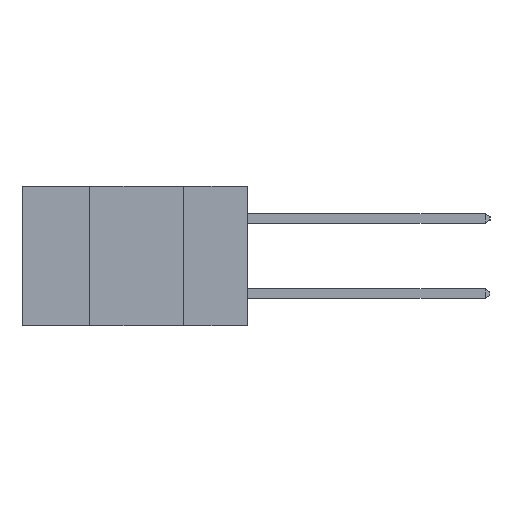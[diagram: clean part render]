
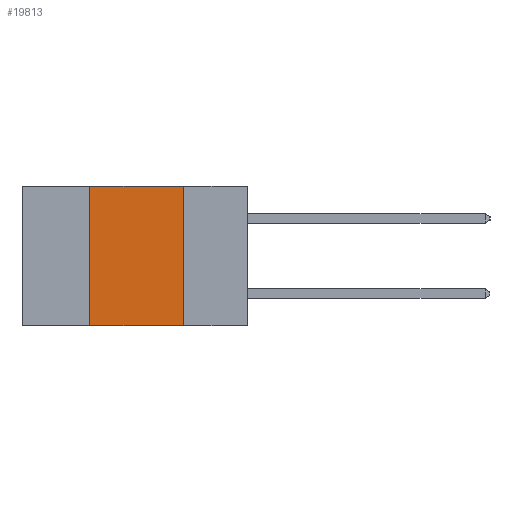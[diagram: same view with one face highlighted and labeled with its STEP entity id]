
A CAD part, left-side view. The second image highlights one B-rep face of the part: STEP entity #19813.
In plain terms, the highlighted planar face has unit normal (-1, 0, 0).
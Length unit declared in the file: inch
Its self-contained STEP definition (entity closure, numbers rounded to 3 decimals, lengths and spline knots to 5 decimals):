
#892 = VECTOR ( 'NONE', #26507, 39.37008 ) ;
#1786 = VERTEX_POINT ( 'NONE', #11524 ) ;
#2100 = DIRECTION ( 'NONE',  ( 0., -1., 0. ) ) ;
#2844 = EDGE_CURVE ( 'NONE', #1786, #5355, #17158, .T. ) ;
#3827 = CARTESIAN_POINT ( 'NONE',  ( 0., 0.6, 0. ) ) ;
#4399 = ORIENTED_EDGE ( 'NONE', *, *, #22895, .F. ) ;
#5173 = LINE ( 'NONE', #23061, #10141 ) ;
#5355 = VERTEX_POINT ( 'NONE', #24916 ) ;
#5968 = DIRECTION ( 'NONE',  ( 0., 0., -1. ) ) ;
#6375 = LINE ( 'NONE', #12646, #11326 ) ;
#7474 = VERTEX_POINT ( 'NONE', #24895 ) ;
#7649 = LINE ( 'NONE', #13156, #18121 ) ;
#9368 = ORIENTED_EDGE ( 'NONE', *, *, #14223, .T. ) ;
#10141 = VECTOR ( 'NONE', #2100, 39.37008 ) ;
#11326 = VECTOR ( 'NONE', #22995, 39.37008 ) ;
#11524 = CARTESIAN_POINT ( 'NONE',  ( 0., 0.17, 0. ) ) ;
#12646 = CARTESIAN_POINT ( 'NONE',  ( 0., 0.6, 0. ) ) ;
#13156 = CARTESIAN_POINT ( 'NONE',  ( 0., 0.42, -0.37 ) ) ;
#14223 = EDGE_CURVE ( 'NONE', #15742, #5355, #5173, .T. ) ;
#15251 = DIRECTION ( 'NONE',  ( 0., 0., 1. ) ) ;
#15742 = VERTEX_POINT ( 'NONE', #19916 ) ;
#17158 = LINE ( 'NONE', #25429, #892 ) ;
#17643 = ORIENTED_EDGE ( 'NONE', *, *, #23748, .F. ) ;
#18060 = EDGE_LOOP ( 'NONE', ( #24440, #4399, #17643, #9368 ) ) ;
#18121 = VECTOR ( 'NONE', #15251, 39.37008 ) ;
#18528 = DIRECTION ( 'NONE',  ( 1., 0., 0. ) ) ;
#19813 = ADVANCED_FACE ( 'NONE', ( #26217 ), #20540, .F. ) ;
#19916 = CARTESIAN_POINT ( 'NONE',  ( 0., 0.42, -0.37 ) ) ;
#20540 = PLANE ( 'NONE',  #25870 ) ;
#22895 = EDGE_CURVE ( 'NONE', #7474, #1786, #6375, .T. ) ;
#22995 = DIRECTION ( 'NONE',  ( 0., -1., 0. ) ) ;
#23061 = CARTESIAN_POINT ( 'NONE',  ( 0., 0.6, -0.37 ) ) ;
#23748 = EDGE_CURVE ( 'NONE', #15742, #7474, #7649, .T. ) ;
#24440 = ORIENTED_EDGE ( 'NONE', *, *, #2844, .F. ) ;
#24895 = CARTESIAN_POINT ( 'NONE',  ( 0., 0.42, 0. ) ) ;
#24916 = CARTESIAN_POINT ( 'NONE',  ( 0., 0.17, -0.37 ) ) ;
#25429 = CARTESIAN_POINT ( 'NONE',  ( 0., 0.17, -0.37 ) ) ;
#25870 = AXIS2_PLACEMENT_3D ( 'NONE', #3827, #18528, #5968 ) ;
#26217 = FACE_OUTER_BOUND ( 'NONE', #18060, .T. ) ;
#26507 = DIRECTION ( 'NONE',  ( 0., 0., -1. ) ) ;
